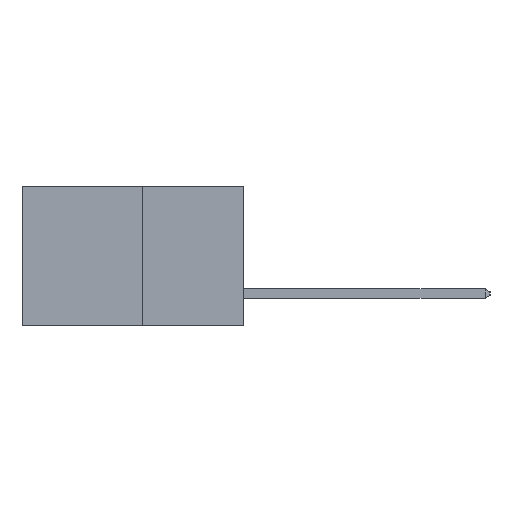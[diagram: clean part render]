
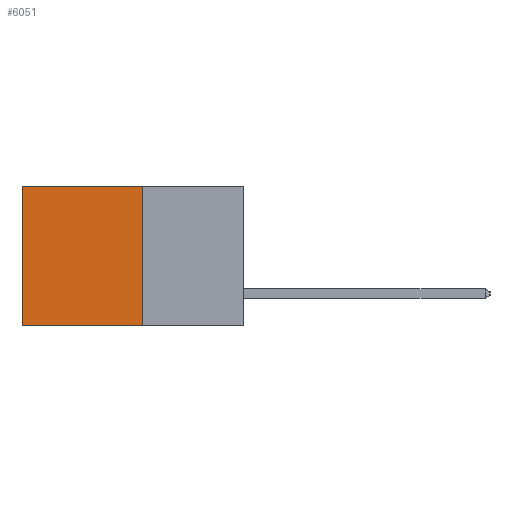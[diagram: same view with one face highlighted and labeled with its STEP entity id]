
A CAD part, left-side view. The second image highlights one B-rep face of the part: STEP entity #6051.
In plain terms, the highlighted planar face has unit normal (-1, 0, 0).
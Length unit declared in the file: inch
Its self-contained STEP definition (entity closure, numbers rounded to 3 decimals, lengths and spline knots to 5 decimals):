
#59 = CARTESIAN_POINT ( 'NONE',  ( 0.277, 0.27, -0.37 ) ) ;
#1328 = VECTOR ( 'NONE', #4006, 39.37008 ) ;
#1341 = ORIENTED_EDGE ( 'NONE', *, *, #16060, .F. ) ;
#2126 = EDGE_CURVE ( 'NONE', #22880, #6711, #21828, .T. ) ;
#2139 = CARTESIAN_POINT ( 'NONE',  ( 0.277, 0.27, -0.37 ) ) ;
#3366 = ORIENTED_EDGE ( 'NONE', *, *, #13034, .T. ) ;
#4006 = DIRECTION ( 'NONE',  ( 0., 1., 0. ) ) ;
#4912 = VERTEX_POINT ( 'NONE', #5287 ) ;
#5287 = CARTESIAN_POINT ( 'NONE',  ( 0.277, 0.59, -0.37 ) ) ;
#5504 = VECTOR ( 'NONE', #13168, 39.37008 ) ;
#6051 = ADVANCED_FACE ( 'NONE', ( #19309 ), #18755, .F. ) ;
#6642 = AXIS2_PLACEMENT_3D ( 'NONE', #18749, #18701, #18676 ) ;
#6711 = VERTEX_POINT ( 'NONE', #8117 ) ;
#7355 = LINE ( 'NONE', #11410, #20465 ) ;
#7709 = ORIENTED_EDGE ( 'NONE', *, *, #10471, .F. ) ;
#8117 = CARTESIAN_POINT ( 'NONE',  ( 0.277, 0.59, 0. ) ) ;
#8678 = CARTESIAN_POINT ( 'NONE',  ( 0.277, 0.27, 0. ) ) ;
#10260 = EDGE_LOOP ( 'NONE', ( #3366, #1341, #7709, #18039 ) ) ;
#10320 = LINE ( 'NONE', #21904, #5504 ) ;
#10471 = EDGE_CURVE ( 'NONE', #22880, #21084, #7355, .T. ) ;
#11410 = CARTESIAN_POINT ( 'NONE',  ( 0.277, 0.27, -0.37 ) ) ;
#11598 = CARTESIAN_POINT ( 'NONE',  ( 0.277, 0.27, 0. ) ) ;
#13034 = EDGE_CURVE ( 'NONE', #6711, #4912, #10320, .T. ) ;
#13168 = DIRECTION ( 'NONE',  ( 0., 0., -1. ) ) ;
#15770 = LINE ( 'NONE', #2139, #1328 ) ;
#16060 = EDGE_CURVE ( 'NONE', #21084, #4912, #15770, .T. ) ;
#17139 = VECTOR ( 'NONE', #19571, 39.37008 ) ;
#18039 = ORIENTED_EDGE ( 'NONE', *, *, #2126, .T. ) ;
#18465 = DIRECTION ( 'NONE',  ( 0., 0., -1. ) ) ;
#18676 = DIRECTION ( 'NONE',  ( 0., 0., -1. ) ) ;
#18701 = DIRECTION ( 'NONE',  ( 1., 0., 0. ) ) ;
#18749 = CARTESIAN_POINT ( 'NONE',  ( 0.277, 0.27, -0.37 ) ) ;
#18755 = PLANE ( 'NONE',  #6642 ) ;
#19309 = FACE_OUTER_BOUND ( 'NONE', #10260, .T. ) ;
#19571 = DIRECTION ( 'NONE',  ( 0., 1., 0. ) ) ;
#20465 = VECTOR ( 'NONE', #18465, 39.37008 ) ;
#21084 = VERTEX_POINT ( 'NONE', #59 ) ;
#21828 = LINE ( 'NONE', #8678, #17139 ) ;
#21904 = CARTESIAN_POINT ( 'NONE',  ( 0.277, 0.59, -0.37 ) ) ;
#22880 = VERTEX_POINT ( 'NONE', #11598 ) ;
